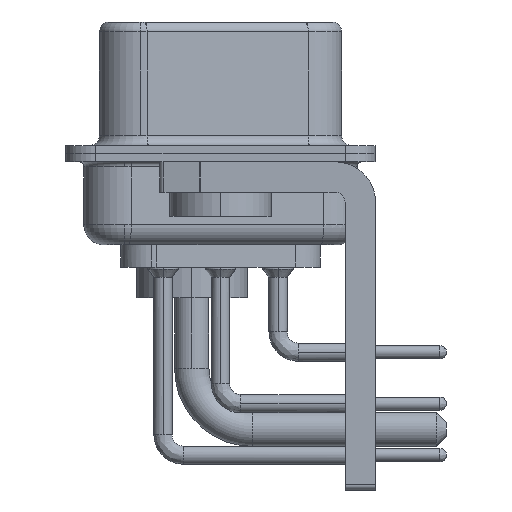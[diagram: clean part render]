
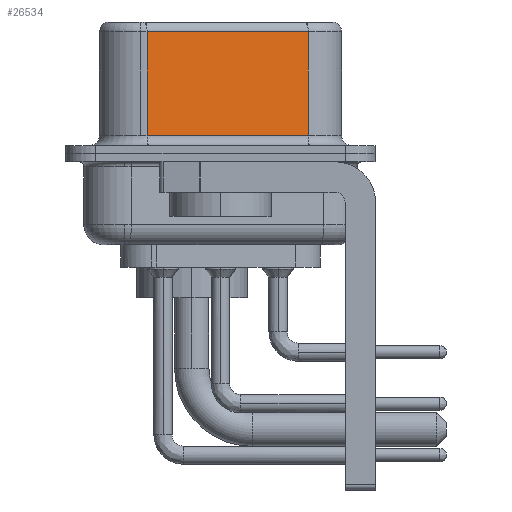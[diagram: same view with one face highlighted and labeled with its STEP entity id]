
A CAD part, left-side view. The second image highlights one B-rep face of the part: STEP entity #26534.
In plain terms, the highlighted planar face has unit normal (-0.985, -0.174, 0).
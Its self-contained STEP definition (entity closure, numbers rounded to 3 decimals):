
#437 = CARTESIAN_POINT ( 'NONE',  ( 5.132, -4.322, 6.52 ) ) ;
#2149 = ORIENTED_EDGE ( 'NONE', *, *, #19214, .F. ) ;
#3710 = DIRECTION ( 'NONE',  ( 0., 0., -1. ) ) ;
#5912 = DIRECTION ( 'NONE',  ( 0.174, -0.985, 0. ) ) ;
#5950 = DIRECTION ( 'NONE',  ( -0.174, 0.985, 0. ) ) ;
#6051 = VECTOR ( 'NONE', #3710, 1000. ) ;
#6529 = CARTESIAN_POINT ( 'NONE',  ( 3.73, 3.628, 6.52 ) ) ;
#8190 = CARTESIAN_POINT ( 'NONE',  ( 5.132, -4.322, 0.9 ) ) ;
#8741 = CARTESIAN_POINT ( 'NONE',  ( 5.132, -4.322, 6.02 ) ) ;
#8920 = LINE ( 'NONE', #8190, #29751 ) ;
#9171 = LINE ( 'NONE', #6529, #6051 ) ;
#9231 = EDGE_LOOP ( 'NONE', ( #2149, #24445, #20763, #23946 ) ) ;
#11381 = CARTESIAN_POINT ( 'NONE',  ( 5.132, -4.322, 0.9 ) ) ;
#11599 = CARTESIAN_POINT ( 'NONE',  ( 5.132, -4.322, 6.02 ) ) ;
#11844 = LINE ( 'NONE', #25921, #34913 ) ;
#11926 = DIRECTION ( 'NONE',  ( 0.985, 0.174, 0. ) ) ;
#14970 = LINE ( 'NONE', #11599, #15574 ) ;
#15120 = PLANE ( 'NONE',  #26823 ) ;
#15574 = VECTOR ( 'NONE', #5950, 1000. ) ;
#19214 = EDGE_CURVE ( 'NONE', #36116, #24547, #11844, .T. ) ;
#20657 = DIRECTION ( 'NONE',  ( 0., 0., -1. ) ) ;
#20705 = CARTESIAN_POINT ( 'NONE',  ( 3.73, 3.628, 0.9 ) ) ;
#20763 = ORIENTED_EDGE ( 'NONE', *, *, #28717, .T. ) ;
#23171 = EDGE_CURVE ( 'NONE', #29168, #24547, #8920, .T. ) ;
#23384 = DIRECTION ( 'NONE',  ( -0.174, 0.985, 0. ) ) ;
#23946 = ORIENTED_EDGE ( 'NONE', *, *, #23171, .T. ) ;
#24445 = ORIENTED_EDGE ( 'NONE', *, *, #34206, .T. ) ;
#24547 = VERTEX_POINT ( 'NONE', #11381 ) ;
#25921 = CARTESIAN_POINT ( 'NONE',  ( 5.132, -4.322, 6.52 ) ) ;
#26534 = ADVANCED_FACE ( 'NONE', ( #29023 ), #15120, .F. ) ;
#26823 = AXIS2_PLACEMENT_3D ( 'NONE', #437, #11926, #23384 ) ;
#28717 = EDGE_CURVE ( 'NONE', #37161, #29168, #9171, .T. ) ;
#29023 = FACE_OUTER_BOUND ( 'NONE', #9231, .T. ) ;
#29168 = VERTEX_POINT ( 'NONE', #20705 ) ;
#29751 = VECTOR ( 'NONE', #5912, 1000. ) ;
#33735 = CARTESIAN_POINT ( 'NONE',  ( 3.73, 3.628, 6.02 ) ) ;
#34206 = EDGE_CURVE ( 'NONE', #36116, #37161, #14970, .T. ) ;
#34913 = VECTOR ( 'NONE', #20657, 1000. ) ;
#36116 = VERTEX_POINT ( 'NONE', #8741 ) ;
#37161 = VERTEX_POINT ( 'NONE', #33735 ) ;
